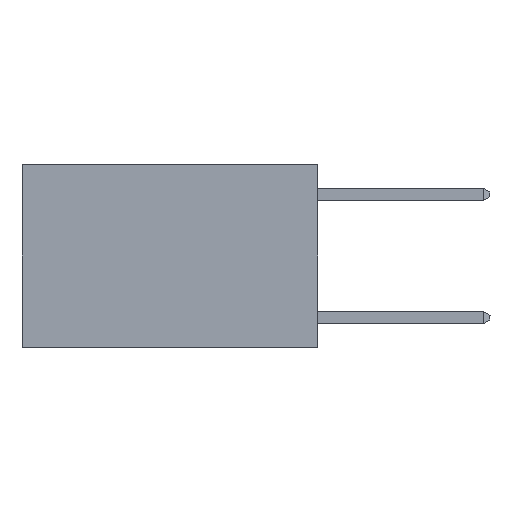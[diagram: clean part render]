
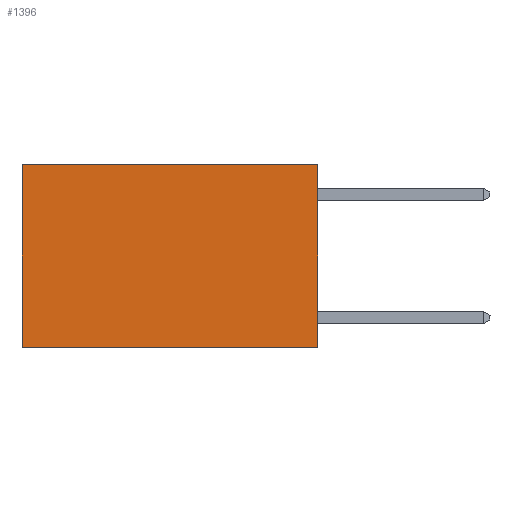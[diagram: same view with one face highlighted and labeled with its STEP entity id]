
A CAD part, left-side view. The second image highlights one B-rep face of the part: STEP entity #1396.
In plain terms, the highlighted planar face has unit normal (-1, 0, 0).
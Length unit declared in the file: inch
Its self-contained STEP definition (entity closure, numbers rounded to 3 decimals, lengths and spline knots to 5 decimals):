
#1114 = PLANE ( 'NONE',  #4355 ) ;
#1396 = ADVANCED_FACE ( 'NONE', ( #13771 ), #1114, .F. ) ;
#1901 = VECTOR ( 'NONE', #12939, 39.37008 ) ;
#2375 = VERTEX_POINT ( 'NONE', #2793 ) ;
#2434 = CARTESIAN_POINT ( 'NONE',  ( 0.2625, 0., 0. ) ) ;
#2746 = VECTOR ( 'NONE', #4067, 39.37008 ) ;
#2793 = CARTESIAN_POINT ( 'NONE',  ( 0.2625, 0., 0. ) ) ;
#3194 = CARTESIAN_POINT ( 'NONE',  ( 0.2625, 0., -0.37 ) ) ;
#4067 = DIRECTION ( 'NONE',  ( 0., 0., -1. ) ) ;
#4262 = ORIENTED_EDGE ( 'NONE', *, *, #20063, .T. ) ;
#4355 = AXIS2_PLACEMENT_3D ( 'NONE', #11316, #8771, #10660 ) ;
#4882 = LINE ( 'NONE', #5590, #17248 ) ;
#5039 = EDGE_CURVE ( 'NONE', #9074, #10206, #14884, .T. ) ;
#5590 = CARTESIAN_POINT ( 'NONE',  ( 0.2625, 0.6, 0. ) ) ;
#6282 = VECTOR ( 'NONE', #17648, 39.37008 ) ;
#6477 = CARTESIAN_POINT ( 'NONE',  ( 0.2625, 0., 0. ) ) ;
#8771 = DIRECTION ( 'NONE',  ( 1., 0., 0. ) ) ;
#9074 = VERTEX_POINT ( 'NONE', #13844 ) ;
#9299 = VERTEX_POINT ( 'NONE', #11232 ) ;
#9720 = EDGE_CURVE ( 'NONE', #2375, #9074, #15707, .T. ) ;
#10206 = VERTEX_POINT ( 'NONE', #14950 ) ;
#10563 = ORIENTED_EDGE ( 'NONE', *, *, #9720, .F. ) ;
#10660 = DIRECTION ( 'NONE',  ( 0., 0., -1. ) ) ;
#11232 = CARTESIAN_POINT ( 'NONE',  ( 0.2625, 0.6, 0. ) ) ;
#11316 = CARTESIAN_POINT ( 'NONE',  ( 0.2625, 0., 0. ) ) ;
#11512 = EDGE_LOOP ( 'NONE', ( #15757, #14871, #10563, #4262 ) ) ;
#12939 = DIRECTION ( 'NONE',  ( 0., 1., 0. ) ) ;
#13771 = FACE_OUTER_BOUND ( 'NONE', #11512, .T. ) ;
#13844 = CARTESIAN_POINT ( 'NONE',  ( 0.2625, 0., -0.37 ) ) ;
#14871 = ORIENTED_EDGE ( 'NONE', *, *, #5039, .F. ) ;
#14884 = LINE ( 'NONE', #3194, #6282 ) ;
#14950 = CARTESIAN_POINT ( 'NONE',  ( 0.2625, 0.6, -0.37 ) ) ;
#15707 = LINE ( 'NONE', #2434, #2746 ) ;
#15757 = ORIENTED_EDGE ( 'NONE', *, *, #17275, .T. ) ;
#17248 = VECTOR ( 'NONE', #18467, 39.37008 ) ;
#17275 = EDGE_CURVE ( 'NONE', #9299, #10206, #4882, .T. ) ;
#17648 = DIRECTION ( 'NONE',  ( 0., 1., 0. ) ) ;
#18467 = DIRECTION ( 'NONE',  ( 0., 0., -1. ) ) ;
#19093 = LINE ( 'NONE', #6477, #1901 ) ;
#20063 = EDGE_CURVE ( 'NONE', #2375, #9299, #19093, .T. ) ;
